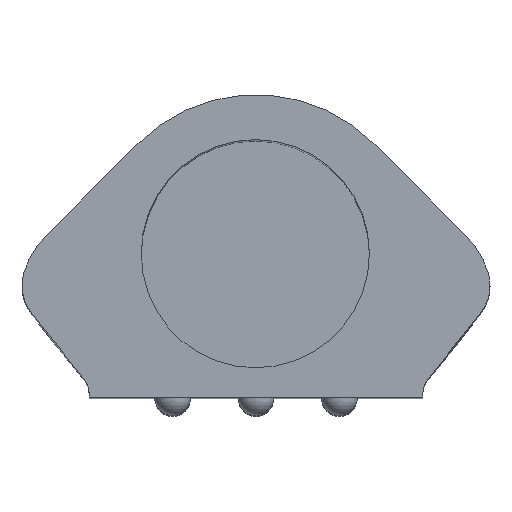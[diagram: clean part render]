
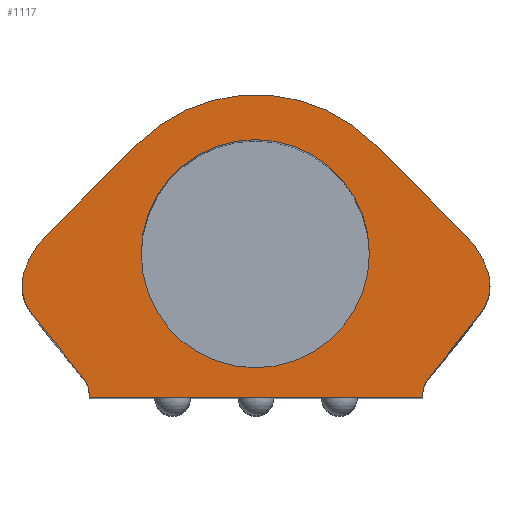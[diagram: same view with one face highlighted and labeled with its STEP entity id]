
A CAD part, top view. The second image highlights one B-rep face of the part: STEP entity #1117.
In plain terms, the highlighted planar face has unit normal (0, 0, 1).
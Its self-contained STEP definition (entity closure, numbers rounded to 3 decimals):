
#2 = EDGE_CURVE ( 'NONE', #496, #62, #1423, .T. ) ;
#5 = ORIENTED_EDGE ( 'NONE', *, *, #1673, .F. ) ;
#10 = DIRECTION ( 'NONE',  ( 0., 0., -1. ) ) ;
#11 = DIRECTION ( 'NONE',  ( 0.624, -0.781, 0. ) ) ;
#24 = VERTEX_POINT ( 'NONE', #451 ) ;
#29 = VERTEX_POINT ( 'NONE', #1685 ) ;
#47 = DIRECTION ( 'NONE',  ( 0., 1., 0. ) ) ;
#48 = VERTEX_POINT ( 'NONE', #846 ) ;
#62 = VERTEX_POINT ( 'NONE', #1119 ) ;
#63 = CARTESIAN_POINT ( 'NONE',  ( -73.897, 62.502, 65.972 ) ) ;
#88 = VERTEX_POINT ( 'NONE', #700 ) ;
#95 = ORIENTED_EDGE ( 'NONE', *, *, #202, .F. ) ;
#104 = CARTESIAN_POINT ( 'NONE',  ( -78.123, 46.473, 65.972 ) ) ;
#107 = CIRCLE ( 'NONE', #312, 5. ) ;
#134 = AXIS2_PLACEMENT_3D ( 'NONE', #616, #298, #1286 ) ;
#137 = AXIS2_PLACEMENT_3D ( 'NONE', #1630, #144, #1494 ) ;
#144 = DIRECTION ( 'NONE',  ( 0., 0., -1. ) ) ;
#147 = CARTESIAN_POINT ( 'NONE',  ( -118.284, 56.904, 65.972 ) ) ;
#154 = EDGE_CURVE ( 'NONE', #783, #1150, #856, .T. ) ;
#180 = EDGE_CURVE ( 'NONE', #1150, #24, #1044, .T. ) ;
#193 = EDGE_CURVE ( 'NONE', #1670, #387, #725, .T. ) ;
#202 = EDGE_CURVE ( 'NONE', #1588, #1735, #107, .T. ) ;
#203 = ORIENTED_EDGE ( 'NONE', *, *, #1104, .F. ) ;
#247 = DIRECTION ( 'NONE',  ( 1., 0., 0. ) ) ;
#249 = VECTOR ( 'NONE', #796, 1000. ) ;
#253 = LINE ( 'NONE', #1561, #1254 ) ;
#258 = EDGE_CURVE ( 'NONE', #695, #1356, #1643, .T. ) ;
#261 = PLANE ( 'NONE',  #1490 ) ;
#273 = CARTESIAN_POINT ( 'NONE',  ( -122.19, 53.784, 65.972 ) ) ;
#276 = AXIS2_PLACEMENT_3D ( 'NONE', #1737, #781, #1594 ) ;
#278 = EDGE_CURVE ( 'NONE', #48, #29, #253, .T. ) ;
#290 = VERTEX_POINT ( 'NONE', #752 ) ;
#292 = DIRECTION ( 'NONE',  ( 1., 0., 0. ) ) ;
#298 = DIRECTION ( 'NONE',  ( 0., 0., -1. ) ) ;
#312 = AXIS2_PLACEMENT_3D ( 'NONE', #770, #1186, #247 ) ;
#335 = AXIS2_PLACEMENT_3D ( 'NONE', #564, #1111, #292 ) ;
#342 = ORIENTED_EDGE ( 'NONE', *, *, #779, .T. ) ;
#355 = ORIENTED_EDGE ( 'NONE', *, *, #154, .T. ) ;
#356 = DIRECTION ( 'NONE',  ( 0.707, -0.707, 0. ) ) ;
#387 = VERTEX_POINT ( 'NONE', #591 ) ;
#394 = VECTOR ( 'NONE', #47, 1000. ) ;
#397 = CARTESIAN_POINT ( 'NONE',  ( -72.283, 53.784, 65.972 ) ) ;
#407 = CARTESIAN_POINT ( 'NONE',  ( -116.35, 46.473, 65.972 ) ) ;
#421 = CARTESIAN_POINT ( 'NONE',  ( -78.67, 32.37, 65.972 ) ) ;
#451 = CARTESIAN_POINT ( 'NONE',  ( -78.123, 46.473, 65.972 ) ) ;
#467 = DIRECTION ( 'NONE',  ( 1., 0., 0. ) ) ;
#496 = VERTEX_POINT ( 'NONE', #962 ) ;
#520 = DIRECTION ( 'NONE',  ( 0., 0., -1. ) ) ;
#535 = CARTESIAN_POINT ( 'NONE',  ( 372.81, 44.49, 65.972 ) ) ;
#542 = CIRCLE ( 'NONE', #335, 2.5 ) ;
#550 = AXIS2_PLACEMENT_3D ( 'NONE', #1439, #1715, #1307 ) ;
#564 = CARTESIAN_POINT ( 'NONE',  ( -118.303, 44.913, 65.972 ) ) ;
#591 = CARTESIAN_POINT ( 'NONE',  ( -116.35, 46.473, 65.972 ) ) ;
#600 = FACE_BOUND ( 'NONE', #1431, .T. ) ;
#601 = CARTESIAN_POINT ( 'NONE',  ( -115.803, 32.37, 65.972 ) ) ;
#616 = CARTESIAN_POINT ( 'NONE',  ( -97.237, 59.573, 65.972 ) ) ;
#659 = DIRECTION ( 'NONE',  ( 0., 0., 1. ) ) ;
#674 = DIRECTION ( 'NONE',  ( 0., 0., -1. ) ) ;
#695 = VERTEX_POINT ( 'NONE', #1742 ) ;
#697 = EDGE_LOOP ( 'NONE', ( #1567, #342, #95, #995, #1099, #993, #1133, #845, #867, #5, #1160, #755, #1720, #203, #355 ) ) ;
#700 = CARTESIAN_POINT ( 'NONE',  ( -97.313, 47.754, 65.972 ) ) ;
#707 = EDGE_CURVE ( 'NONE', #1054, #88, #1193, .T. ) ;
#725 = LINE ( 'NONE', #407, #1089 ) ;
#729 = CARTESIAN_POINT ( 'NONE',  ( -71.19, 56.904, 65.972 ) ) ;
#752 = CARTESIAN_POINT ( 'NONE',  ( -71.412, 58.378, 65.972 ) ) ;
#755 = ORIENTED_EDGE ( 'NONE', *, *, #1537, .T. ) ;
#770 = CARTESIAN_POINT ( 'NONE',  ( -76.19, 56.904, 65.972 ) ) ;
#778 = DIRECTION ( 'NONE',  ( 1., 0., 0. ) ) ;
#779 = EDGE_CURVE ( 'NONE', #24, #1735, #1023, .T. ) ;
#781 = DIRECTION ( 'NONE',  ( 0., 0., -1. ) ) ;
#783 = VERTEX_POINT ( 'NONE', #1304 ) ;
#790 = CARTESIAN_POINT ( 'NONE',  ( 210.223, 23.523, 65.972 ) ) ;
#796 = DIRECTION ( 'NONE',  ( -1., 0., 0. ) ) ;
#809 = DIRECTION ( 'NONE',  ( 1., 0., 0. ) ) ;
#819 = CARTESIAN_POINT ( 'NONE',  ( -97.313, 73.154, 65.972 ) ) ;
#845 = ORIENTED_EDGE ( 'NONE', *, *, #278, .F. ) ;
#846 = CARTESIAN_POINT ( 'NONE',  ( -120.577, 62.502, 65.972 ) ) ;
#856 = LINE ( 'NONE', #421, #1575 ) ;
#867 = ORIENTED_EDGE ( 'NONE', *, *, #1225, .F. ) ;
#897 = CARTESIAN_POINT ( 'NONE',  ( -84.102, 72.707, 65.972 ) ) ;
#918 = VECTOR ( 'NONE', #356, 1000. ) ;
#924 = CARTESIAN_POINT ( 'NONE',  ( -78.67, 44.913, 65.972 ) ) ;
#946 = AXIS2_PLACEMENT_3D ( 'NONE', #1543, #1401, #467 ) ;
#953 = EDGE_CURVE ( 'NONE', #29, #695, #1615, .T. ) ;
#962 = CARTESIAN_POINT ( 'NONE',  ( -115.803, 44.49, 65.972 ) ) ;
#993 = ORIENTED_EDGE ( 'NONE', *, *, #258, .F. ) ;
#995 = ORIENTED_EDGE ( 'NONE', *, *, #1052, .F. ) ;
#1023 = LINE ( 'NONE', #104, #1706 ) ;
#1035 = DIRECTION ( 'NONE',  ( 0.624, 0.781, 0. ) ) ;
#1038 = CIRCLE ( 'NONE', #946, 10. ) ;
#1040 = CIRCLE ( 'NONE', #137, 5. ) ;
#1044 = CIRCLE ( 'NONE', #1121, 2.5 ) ;
#1051 = CARTESIAN_POINT ( 'NONE',  ( -97.313, 60.454, 65.972 ) ) ;
#1052 = EDGE_CURVE ( 'NONE', #290, #1588, #1040, .T. ) ;
#1054 = VERTEX_POINT ( 'NONE', #819 ) ;
#1089 = VECTOR ( 'NONE', #11, 1000. ) ;
#1091 = DIRECTION ( 'NONE',  ( 0., 1., 0. ) ) ;
#1099 = ORIENTED_EDGE ( 'NONE', *, *, #1637, .F. ) ;
#1104 = EDGE_CURVE ( 'NONE', #783, #496, #1359, .T. ) ;
#1111 = DIRECTION ( 'NONE',  ( 0., 0., -1. ) ) ;
#1117 = ADVANCED_FACE ( 'NONE', ( #1638, #600 ), #261, .T. ) ;
#1119 = CARTESIAN_POINT ( 'NONE',  ( -115.803, 44.913, 65.972 ) ) ;
#1121 = AXIS2_PLACEMENT_3D ( 'NONE', #1627, #674, #1488 ) ;
#1133 = ORIENTED_EDGE ( 'NONE', *, *, #953, .F. ) ;
#1146 = CIRCLE ( 'NONE', #550, 10. ) ;
#1150 = VERTEX_POINT ( 'NONE', #924 ) ;
#1155 = EDGE_CURVE ( 'NONE', #88, #1054, #1275, .T. ) ;
#1160 = ORIENTED_EDGE ( 'NONE', *, *, #193, .T. ) ;
#1171 = AXIS2_PLACEMENT_3D ( 'NONE', #147, #10, #809 ) ;
#1186 = DIRECTION ( 'NONE',  ( 0., 0., -1. ) ) ;
#1193 = CIRCLE ( 'NONE', #276, 12.7 ) ;
#1225 = EDGE_CURVE ( 'NONE', #1311, #48, #1146, .T. ) ;
#1254 = VECTOR ( 'NONE', #1295, 1000. ) ;
#1275 = CIRCLE ( 'NONE', #1395, 12.7 ) ;
#1286 = DIRECTION ( 'NONE',  ( 1., 0., 0. ) ) ;
#1295 = DIRECTION ( 'NONE',  ( 0.707, 0.707, 0. ) ) ;
#1304 = CARTESIAN_POINT ( 'NONE',  ( -78.67, 44.49, 65.972 ) ) ;
#1307 = DIRECTION ( 'NONE',  ( 1., 0., 0. ) ) ;
#1311 = VERTEX_POINT ( 'NONE', #1566 ) ;
#1356 = VERTEX_POINT ( 'NONE', #63 ) ;
#1359 = LINE ( 'NONE', #535, #249 ) ;
#1395 = AXIS2_PLACEMENT_3D ( 'NONE', #1051, #520, #778 ) ;
#1401 = DIRECTION ( 'NONE',  ( 0., 0., -1. ) ) ;
#1423 = LINE ( 'NONE', #601, #394 ) ;
#1425 = ORIENTED_EDGE ( 'NONE', *, *, #707, .T. ) ;
#1431 = EDGE_LOOP ( 'NONE', ( #1425, #1549 ) ) ;
#1439 = CARTESIAN_POINT ( 'NONE',  ( -113.506, 55.43, 65.972 ) ) ;
#1488 = DIRECTION ( 'NONE',  ( 1., 0., 0. ) ) ;
#1490 = AXIS2_PLACEMENT_3D ( 'NONE', #790, #659, #1744 ) ;
#1494 = DIRECTION ( 'NONE',  ( 1., 0., 0. ) ) ;
#1537 = EDGE_CURVE ( 'NONE', #387, #62, #542, .T. ) ;
#1543 = CARTESIAN_POINT ( 'NONE',  ( -80.968, 55.43, 65.972 ) ) ;
#1549 = ORIENTED_EDGE ( 'NONE', *, *, #1155, .T. ) ;
#1561 = CARTESIAN_POINT ( 'NONE',  ( -110.371, 72.707, 65.972 ) ) ;
#1566 = CARTESIAN_POINT ( 'NONE',  ( -123.061, 58.378, 65.972 ) ) ;
#1567 = ORIENTED_EDGE ( 'NONE', *, *, #180, .T. ) ;
#1575 = VECTOR ( 'NONE', #1091, 1000. ) ;
#1588 = VERTEX_POINT ( 'NONE', #729 ) ;
#1594 = DIRECTION ( 'NONE',  ( 1., 0., 0. ) ) ;
#1615 = CIRCLE ( 'NONE', #134, 18.575 ) ;
#1627 = CARTESIAN_POINT ( 'NONE',  ( -76.17, 44.913, 65.972 ) ) ;
#1630 = CARTESIAN_POINT ( 'NONE',  ( -76.19, 56.904, 65.972 ) ) ;
#1637 = EDGE_CURVE ( 'NONE', #1356, #290, #1038, .T. ) ;
#1638 = FACE_OUTER_BOUND ( 'NONE', #697, .T. ) ;
#1643 = LINE ( 'NONE', #897, #918 ) ;
#1670 = VERTEX_POINT ( 'NONE', #273 ) ;
#1673 = EDGE_CURVE ( 'NONE', #1670, #1311, #1713, .T. ) ;
#1685 = CARTESIAN_POINT ( 'NONE',  ( -110.371, 72.707, 65.972 ) ) ;
#1706 = VECTOR ( 'NONE', #1035, 1000. ) ;
#1713 = CIRCLE ( 'NONE', #1171, 5. ) ;
#1715 = DIRECTION ( 'NONE',  ( 0., 0., -1. ) ) ;
#1720 = ORIENTED_EDGE ( 'NONE', *, *, #2, .F. ) ;
#1735 = VERTEX_POINT ( 'NONE', #397 ) ;
#1737 = CARTESIAN_POINT ( 'NONE',  ( -97.313, 60.454, 65.972 ) ) ;
#1742 = CARTESIAN_POINT ( 'NONE',  ( -84.102, 72.707, 65.972 ) ) ;
#1744 = DIRECTION ( 'NONE',  ( 1., 0., 0. ) ) ;
